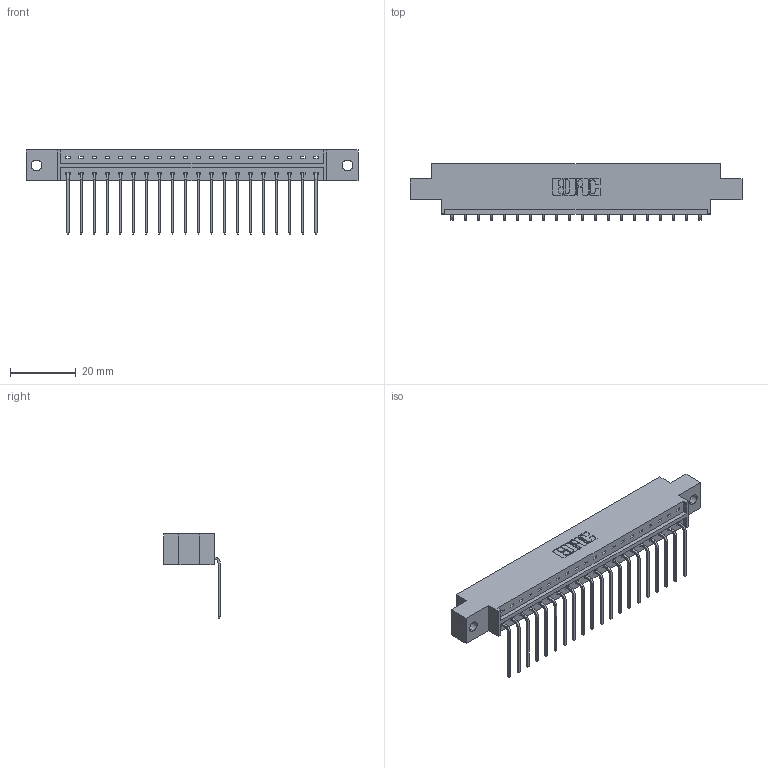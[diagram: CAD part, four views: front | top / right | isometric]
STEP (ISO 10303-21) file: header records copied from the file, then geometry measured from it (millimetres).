
FILE_DESCRIPTION (( 'STEP AP203' ), '1' );
FILE_NAME ('833-020-559-602.STEP', '2020-06-01T14:12:15', ( '' ), ( '' ), 'SwSTEP 2.0', 'SolidWorks 2020', '' );
FILE_SCHEMA (( 'CONFIG_CONTROL_DESIGN' ));
Length unit declared in the file: inch
Products named in the file (3): 345-292-001_558 559 Tail - 1; 833 Part_Offset - .128 Dia; 833-020-559-602
Assembly tree (21 placements, depth 2):
  833-020-559-602
    833 Part_Offset - .128 Dia
    345-292-001_558 559 Tail - 1  x20
Bounding box: 100.79 x 17.09 x 25.53 mm (x, y, z)
Volume: 9755 mm3; surface area: 10745.1 mm2
Topology: 21 solids, 21 shells, 1318 faces, 3963 edges, 2614 vertices
Faces by surface type: plane 954, cylinder 364
Entity records: 15291 total; most frequent: CARTESIAN_POINT 2650, ORIENTED_EDGE 2606, DIRECTION 2279, EDGE_CURVE 1303, VECTOR 1175, LINE 1175, VERTEX_POINT 866, AXIS2_PLACEMENT_3D 552
